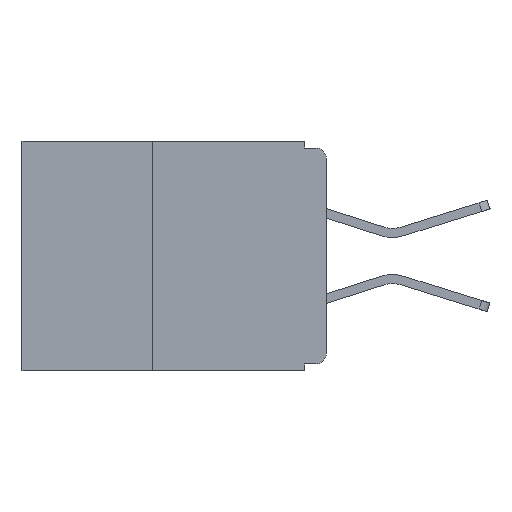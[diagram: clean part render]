
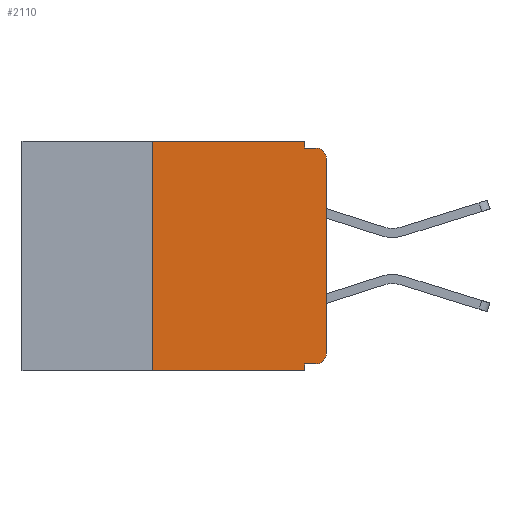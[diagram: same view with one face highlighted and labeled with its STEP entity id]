
A CAD part, left-side view. The second image highlights one B-rep face of the part: STEP entity #2110.
In plain terms, the highlighted planar face has unit normal (-1, 0, 0).
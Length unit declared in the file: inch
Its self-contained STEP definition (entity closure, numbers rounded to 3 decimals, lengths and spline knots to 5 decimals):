
#48 = CARTESIAN_POINT ( 'NONE',  ( 0., 0., -0.01 ) ) ;
#393 = ORIENTED_EDGE ( 'NONE', *, *, #1841, .F. ) ;
#488 = LINE ( 'NONE', #10330, #11499 ) ;
#807 = EDGE_LOOP ( 'NONE', ( #3614, #1501, #2895, #1807, #9907, #393, #2499, #2982, #3816, #5268 ) ) ;
#895 = VERTEX_POINT ( 'NONE', #908 ) ;
#908 = CARTESIAN_POINT ( 'NONE',  ( 0., 0., -0.025 ) ) ;
#1041 = CARTESIAN_POINT ( 'NONE',  ( 0., 0.25, -0.33 ) ) ;
#1152 = AXIS2_PLACEMENT_3D ( 'NONE', #10711, #11780, #7561 ) ;
#1501 = ORIENTED_EDGE ( 'NONE', *, *, #9716, .T. ) ;
#1807 = ORIENTED_EDGE ( 'NONE', *, *, #3341, .F. ) ;
#1841 = EDGE_CURVE ( 'NONE', #2504, #12082, #3174, .T. ) ;
#2110 = ADVANCED_FACE ( 'NONE', ( #5474 ), #8821, .F. ) ;
#2499 = ORIENTED_EDGE ( 'NONE', *, *, #6600, .T. ) ;
#2504 = VERTEX_POINT ( 'NONE', #1041 ) ;
#2895 = ORIENTED_EDGE ( 'NONE', *, *, #6003, .F. ) ;
#2982 = ORIENTED_EDGE ( 'NONE', *, *, #5280, .F. ) ;
#3006 = VERTEX_POINT ( 'NONE', #11343 ) ;
#3174 = LINE ( 'NONE', #6054, #5652 ) ;
#3341 = EDGE_CURVE ( 'NONE', #4998, #11135, #8968, .T. ) ;
#3363 = CARTESIAN_POINT ( 'NONE',  ( 0., 0.015, -0.305 ) ) ;
#3386 = VECTOR ( 'NONE', #9509, 39.37008 ) ;
#3575 = CARTESIAN_POINT ( 'NONE',  ( 0., 0.437, 0. ) ) ;
#3614 = ORIENTED_EDGE ( 'NONE', *, *, #8872, .T. ) ;
#3659 = DIRECTION ( 'NONE',  ( 0., -1., 0. ) ) ;
#3716 = LINE ( 'NONE', #9615, #3386 ) ;
#3816 = ORIENTED_EDGE ( 'NONE', *, *, #9459, .F. ) ;
#3947 = VERTEX_POINT ( 'NONE', #8617 ) ;
#4322 = DIRECTION ( 'NONE',  ( 0., 0., -1. ) ) ;
#4334 = DIRECTION ( 'NONE',  ( -1., 0., 0. ) ) ;
#4345 = CARTESIAN_POINT ( 'NONE',  ( 0., 0.015, -0.025 ) ) ;
#4440 = DIRECTION ( 'NONE',  ( 0., 0., -1. ) ) ;
#4725 = VECTOR ( 'NONE', #5877, 39.37008 ) ;
#4998 = VERTEX_POINT ( 'NONE', #5658 ) ;
#5268 = ORIENTED_EDGE ( 'NONE', *, *, #11648, .T. ) ;
#5280 = EDGE_CURVE ( 'NONE', #8660, #3947, #11393, .T. ) ;
#5308 = VECTOR ( 'NONE', #3659, 39.37008 ) ;
#5474 = FACE_OUTER_BOUND ( 'NONE', #807, .T. ) ;
#5652 = VECTOR ( 'NONE', #10398, 39.37008 ) ;
#5658 = CARTESIAN_POINT ( 'NONE',  ( 0., 0.031, 0. ) ) ;
#5778 = VECTOR ( 'NONE', #13143, 39.37008 ) ;
#5827 = EDGE_CURVE ( 'NONE', #12082, #4998, #10622, .T. ) ;
#5864 = CARTESIAN_POINT ( 'NONE',  ( 0., 0., -0.32 ) ) ;
#5877 = DIRECTION ( 'NONE',  ( 0., 1., 0. ) ) ;
#6003 = EDGE_CURVE ( 'NONE', #11135, #3006, #11089, .T. ) ;
#6054 = CARTESIAN_POINT ( 'NONE',  ( 0., 0.25, -0.33 ) ) ;
#6278 = VECTOR ( 'NONE', #11536, 39.37008 ) ;
#6533 = CARTESIAN_POINT ( 'NONE',  ( 0., 0.015, -0.32 ) ) ;
#6552 = CARTESIAN_POINT ( 'NONE',  ( 0., 0.031, -0.01 ) ) ;
#6560 = AXIS2_PLACEMENT_3D ( 'NONE', #4345, #4334, #4322 ) ;
#6600 = EDGE_CURVE ( 'NONE', #2504, #3947, #488, .T. ) ;
#7134 = CARTESIAN_POINT ( 'NONE',  ( 0., 0.25, 0. ) ) ;
#7561 = DIRECTION ( 'NONE',  ( 0., 0., -1. ) ) ;
#8601 = VERTEX_POINT ( 'NONE', #11292 ) ;
#8617 = CARTESIAN_POINT ( 'NONE',  ( 0., 0.031, -0.33 ) ) ;
#8660 = VERTEX_POINT ( 'NONE', #10894 ) ;
#8821 = PLANE ( 'NONE',  #1152 ) ;
#8872 = EDGE_CURVE ( 'NONE', #8601, #895, #3716, .T. ) ;
#8968 = LINE ( 'NONE', #12627, #6278 ) ;
#9062 = CIRCLE ( 'NONE', #12776, 0.015 ) ;
#9282 = CIRCLE ( 'NONE', #6560, 0.015 ) ;
#9351 = VERTEX_POINT ( 'NONE', #6533 ) ;
#9459 = EDGE_CURVE ( 'NONE', #9351, #8660, #12316, .T. ) ;
#9509 = DIRECTION ( 'NONE',  ( 0., 0., 1. ) ) ;
#9615 = CARTESIAN_POINT ( 'NONE',  ( 0., 0., 0. ) ) ;
#9716 = EDGE_CURVE ( 'NONE', #895, #3006, #9282, .T. ) ;
#9907 = ORIENTED_EDGE ( 'NONE', *, *, #5827, .F. ) ;
#10172 = VECTOR ( 'NONE', #11396, 39.37008 ) ;
#10330 = CARTESIAN_POINT ( 'NONE',  ( 0., 0.437, -0.33 ) ) ;
#10398 = DIRECTION ( 'NONE',  ( 0., 0., 1. ) ) ;
#10425 = DIRECTION ( 'NONE',  ( 0., -1., 0. ) ) ;
#10453 = DIRECTION ( 'NONE',  ( -1., 0., 0. ) ) ;
#10622 = LINE ( 'NONE', #3575, #5308 ) ;
#10711 = CARTESIAN_POINT ( 'NONE',  ( 0., 0.437, 0. ) ) ;
#10894 = CARTESIAN_POINT ( 'NONE',  ( 0., 0.031, -0.32 ) ) ;
#11089 = LINE ( 'NONE', #48, #5778 ) ;
#11135 = VERTEX_POINT ( 'NONE', #6552 ) ;
#11292 = CARTESIAN_POINT ( 'NONE',  ( 0., 0., -0.305 ) ) ;
#11343 = CARTESIAN_POINT ( 'NONE',  ( 0., 0.015, -0.01 ) ) ;
#11393 = LINE ( 'NONE', #11484, #10172 ) ;
#11396 = DIRECTION ( 'NONE',  ( 0., 0., -1. ) ) ;
#11484 = CARTESIAN_POINT ( 'NONE',  ( 0., 0.031, -0.33 ) ) ;
#11499 = VECTOR ( 'NONE', #10425, 39.37008 ) ;
#11536 = DIRECTION ( 'NONE',  ( 0., 0., -1. ) ) ;
#11648 = EDGE_CURVE ( 'NONE', #9351, #8601, #9062, .T. ) ;
#11780 = DIRECTION ( 'NONE',  ( 1., 0., 0. ) ) ;
#12082 = VERTEX_POINT ( 'NONE', #7134 ) ;
#12316 = LINE ( 'NONE', #5864, #4725 ) ;
#12627 = CARTESIAN_POINT ( 'NONE',  ( 0., 0.031, 0. ) ) ;
#12776 = AXIS2_PLACEMENT_3D ( 'NONE', #3363, #10453, #4440 ) ;
#13143 = DIRECTION ( 'NONE',  ( 0., -1., 0. ) ) ;
